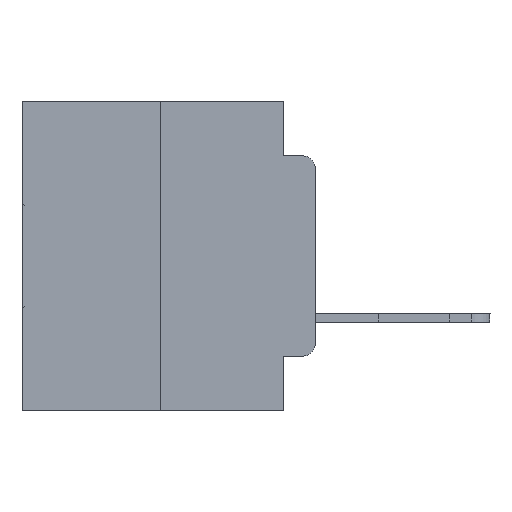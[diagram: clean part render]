
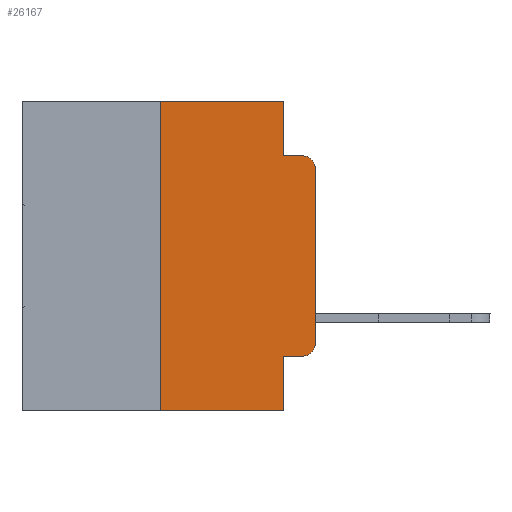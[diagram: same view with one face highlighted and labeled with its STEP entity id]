
A CAD part, left-side view. The second image highlights one B-rep face of the part: STEP entity #26167.
In plain terms, the highlighted planar face has unit normal (-1, 0, 0).
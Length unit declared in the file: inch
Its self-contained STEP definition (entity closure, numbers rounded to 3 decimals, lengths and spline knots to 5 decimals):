
#295 = ORIENTED_EDGE ( 'NONE', *, *, #4603, .T. ) ;
#623 = EDGE_CURVE ( 'NONE', #3747, #1644, #17968, .T. ) ;
#643 = CARTESIAN_POINT ( 'NONE',  ( 0., 0., -0.3915 ) ) ;
#883 = ORIENTED_EDGE ( 'NONE', *, *, #23762, .F. ) ;
#970 = AXIS2_PLACEMENT_3D ( 'NONE', #20326, #15617, #27005 ) ;
#1329 = VECTOR ( 'NONE', #29343, 39.37008 ) ;
#1393 = CARTESIAN_POINT ( 'NONE',  ( 0., 0., 0. ) ) ;
#1644 = VERTEX_POINT ( 'NONE', #11601 ) ;
#2073 = CARTESIAN_POINT ( 'NONE',  ( 0., 0., -0.1085 ) ) ;
#2179 = CARTESIAN_POINT ( 'NONE',  ( 0., 0.051, -0.0885 ) ) ;
#2851 = LINE ( 'NONE', #9878, #26793 ) ;
#2883 = VECTOR ( 'NONE', #10648, 39.37008 ) ;
#3747 = VERTEX_POINT ( 'NONE', #9547 ) ;
#3841 = EDGE_CURVE ( 'NONE', #29165, #28948, #28425, .T. ) ;
#3910 = DIRECTION ( 'NONE',  ( 0., -1., 0. ) ) ;
#4165 = EDGE_CURVE ( 'NONE', #28948, #14726, #9135, .T. ) ;
#4571 = EDGE_CURVE ( 'NONE', #8078, #24028, #14004, .T. ) ;
#4603 = EDGE_CURVE ( 'NONE', #24028, #29165, #29087, .T. ) ;
#5174 = ORIENTED_EDGE ( 'NONE', *, *, #7122, .F. ) ;
#6187 = LINE ( 'NONE', #20071, #1329 ) ;
#7035 = DIRECTION ( 'NONE',  ( -1., 0., 0. ) ) ;
#7122 = EDGE_CURVE ( 'NONE', #1644, #7180, #2851, .T. ) ;
#7180 = VERTEX_POINT ( 'NONE', #17325 ) ;
#7313 = DIRECTION ( 'NONE',  ( 0., 0., -1. ) ) ;
#8078 = VERTEX_POINT ( 'NONE', #24264 ) ;
#9031 = EDGE_CURVE ( 'NONE', #27389, #14726, #29506, .T. ) ;
#9135 = CIRCLE ( 'NONE', #27117, 0.02 ) ;
#9481 = DIRECTION ( 'NONE',  ( -1., 0., 0. ) ) ;
#9547 = CARTESIAN_POINT ( 'NONE',  ( 0., 0.25, -0.5 ) ) ;
#9779 = ORIENTED_EDGE ( 'NONE', *, *, #17937, .F. ) ;
#9878 = CARTESIAN_POINT ( 'NONE',  ( 0., 0.473, 0. ) ) ;
#10648 = DIRECTION ( 'NONE',  ( 0., 0., 1. ) ) ;
#11399 = LINE ( 'NONE', #20692, #12120 ) ;
#11601 = CARTESIAN_POINT ( 'NONE',  ( 0., 0.25, 0. ) ) ;
#11918 = DIRECTION ( 'NONE',  ( 0., 0., -1. ) ) ;
#12120 = VECTOR ( 'NONE', #29967, 39.37008 ) ;
#13169 = ORIENTED_EDGE ( 'NONE', *, *, #623, .F. ) ;
#14004 = LINE ( 'NONE', #23313, #24267 ) ;
#14710 = CARTESIAN_POINT ( 'NONE',  ( 0., 0.02, -0.0885 ) ) ;
#14726 = VERTEX_POINT ( 'NONE', #14710 ) ;
#15197 = VERTEX_POINT ( 'NONE', #27066 ) ;
#15507 = CARTESIAN_POINT ( 'NONE',  ( 0., 0.051, -0.0885 ) ) ;
#15617 = DIRECTION ( 'NONE',  ( 1., 0., 0. ) ) ;
#16426 = VECTOR ( 'NONE', #27110, 39.37008 ) ;
#16884 = EDGE_LOOP ( 'NONE', ( #27702, #24943, #21370, #9779, #5174, #13169, #25535, #883, #23091, #295 ) ) ;
#17325 = CARTESIAN_POINT ( 'NONE',  ( 0., 0.051, 0. ) ) ;
#17907 = PLANE ( 'NONE',  #970 ) ;
#17937 = EDGE_CURVE ( 'NONE', #7180, #27389, #11399, .T. ) ;
#17968 = LINE ( 'NONE', #24804, #2883 ) ;
#19455 = VECTOR ( 'NONE', #24720, 39.37008 ) ;
#20071 = CARTESIAN_POINT ( 'NONE',  ( 0., 0.051, 0. ) ) ;
#20326 = CARTESIAN_POINT ( 'NONE',  ( 0., 0.473, 0. ) ) ;
#20692 = CARTESIAN_POINT ( 'NONE',  ( 0., 0.051, 0. ) ) ;
#20868 = CARTESIAN_POINT ( 'NONE',  ( 0., 0.02, -0.3915 ) ) ;
#21370 = ORIENTED_EDGE ( 'NONE', *, *, #9031, .F. ) ;
#21540 = EDGE_CURVE ( 'NONE', #3747, #15197, #27724, .T. ) ;
#21730 = CARTESIAN_POINT ( 'NONE',  ( 0., 0.02, -0.4115 ) ) ;
#23091 = ORIENTED_EDGE ( 'NONE', *, *, #4571, .T. ) ;
#23313 = CARTESIAN_POINT ( 'NONE',  ( 0., 0.051, -0.4115 ) ) ;
#23504 = CARTESIAN_POINT ( 'NONE',  ( 0., 0.02, -0.1085 ) ) ;
#23762 = EDGE_CURVE ( 'NONE', #8078, #15197, #6187, .T. ) ;
#24028 = VERTEX_POINT ( 'NONE', #21730 ) ;
#24264 = CARTESIAN_POINT ( 'NONE',  ( 0., 0.051, -0.4115 ) ) ;
#24267 = VECTOR ( 'NONE', #28158, 39.37008 ) ;
#24720 = DIRECTION ( 'NONE',  ( 0., 0., 1. ) ) ;
#24804 = CARTESIAN_POINT ( 'NONE',  ( 0., 0.25, 0. ) ) ;
#24943 = ORIENTED_EDGE ( 'NONE', *, *, #4165, .T. ) ;
#25535 = ORIENTED_EDGE ( 'NONE', *, *, #21540, .T. ) ;
#25703 = AXIS2_PLACEMENT_3D ( 'NONE', #20868, #7035, #7313 ) ;
#26167 = ADVANCED_FACE ( 'NONE', ( #29611 ), #17907, .F. ) ;
#26793 = VECTOR ( 'NONE', #28445, 39.37008 ) ;
#27005 = DIRECTION ( 'NONE',  ( 0., 0., -1. ) ) ;
#27066 = CARTESIAN_POINT ( 'NONE',  ( 0., 0.051, -0.5 ) ) ;
#27110 = DIRECTION ( 'NONE',  ( 0., -1., 0. ) ) ;
#27117 = AXIS2_PLACEMENT_3D ( 'NONE', #23504, #9481, #11918 ) ;
#27389 = VERTEX_POINT ( 'NONE', #2179 ) ;
#27702 = ORIENTED_EDGE ( 'NONE', *, *, #3841, .T. ) ;
#27724 = LINE ( 'NONE', #30012, #16426 ) ;
#27855 = VECTOR ( 'NONE', #3910, 39.37008 ) ;
#28158 = DIRECTION ( 'NONE',  ( 0., -1., 0. ) ) ;
#28425 = LINE ( 'NONE', #1393, #19455 ) ;
#28445 = DIRECTION ( 'NONE',  ( 0., -1., 0. ) ) ;
#28948 = VERTEX_POINT ( 'NONE', #2073 ) ;
#29087 = CIRCLE ( 'NONE', #25703, 0.02 ) ;
#29165 = VERTEX_POINT ( 'NONE', #643 ) ;
#29343 = DIRECTION ( 'NONE',  ( 0., 0., -1. ) ) ;
#29506 = LINE ( 'NONE', #15507, #27855 ) ;
#29611 = FACE_OUTER_BOUND ( 'NONE', #16884, .T. ) ;
#29967 = DIRECTION ( 'NONE',  ( 0., 0., -1. ) ) ;
#30012 = CARTESIAN_POINT ( 'NONE',  ( 0., 0.473, -0.5 ) ) ;
